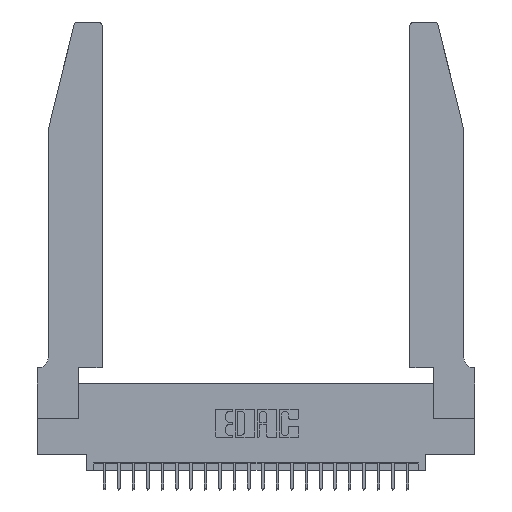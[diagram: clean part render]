
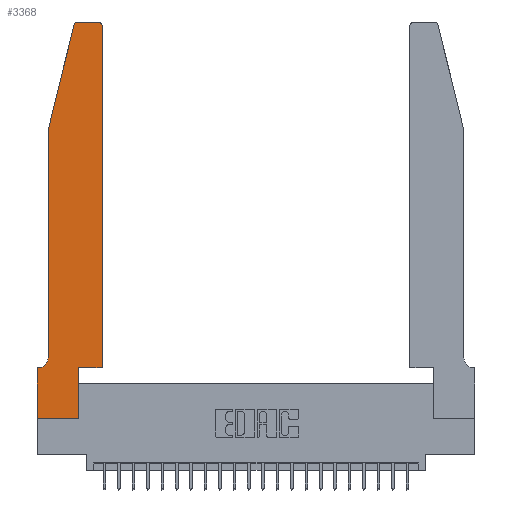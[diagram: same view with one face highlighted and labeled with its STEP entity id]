
A CAD part, top view. The second image highlights one B-rep face of the part: STEP entity #3368.
In plain terms, the highlighted planar face has unit normal (0, 0, 1).
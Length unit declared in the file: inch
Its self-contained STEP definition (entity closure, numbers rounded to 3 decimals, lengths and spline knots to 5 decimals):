
#130 = DIRECTION ( 'NONE',  ( -0.239, -0.971, 0. ) ) ;
#488 = CARTESIAN_POINT ( 'NONE',  ( 0.0755, 2., 0.37 ) ) ;
#593 = EDGE_CURVE ( 'NONE', #7490, #12814, #12112, .T. ) ;
#648 = DIRECTION ( 'NONE',  ( 1., 0., 0. ) ) ;
#913 = EDGE_CURVE ( 'NONE', #7336, #8099, #11092, .T. ) ;
#1111 = DIRECTION ( 'NONE',  ( 0., 0., 1. ) ) ;
#1281 = CARTESIAN_POINT ( 'NONE',  ( 0.0755, 0.42, 0.37 ) ) ;
#1291 = ORIENTED_EDGE ( 'NONE', *, *, #3324, .T. ) ;
#1576 = ORIENTED_EDGE ( 'NONE', *, *, #6813, .T. ) ;
#1815 = CIRCLE ( 'NONE', #7469, 0.07 ) ;
#1848 = ORIENTED_EDGE ( 'NONE', *, *, #8967, .T. ) ;
#2276 = VERTEX_POINT ( 'NONE', #1281 ) ;
#2539 = CARTESIAN_POINT ( 'NONE',  ( 0.2605, 2.75, 0.37 ) ) ;
#2674 = DIRECTION ( 'NONE',  ( -1., 0., 0. ) ) ;
#2906 = CIRCLE ( 'NONE', #4933, 0.03 ) ;
#3324 = EDGE_CURVE ( 'NONE', #22680, #20967, #6829, .T. ) ;
#3368 = ADVANCED_FACE ( 'NONE', ( #19996 ), #8461, .T. ) ;
#3487 = LINE ( 'NONE', #17595, #19776 ) ;
#3553 = DIRECTION ( 'NONE',  ( 0., 0., 1. ) ) ;
#4190 = EDGE_CURVE ( 'NONE', #8099, #7490, #8575, .T. ) ;
#4331 = CARTESIAN_POINT ( 'NONE',  ( 0.284, 2.75, 0.37 ) ) ;
#4577 = VECTOR ( 'NONE', #10924, 39.37008 ) ;
#4749 = CARTESIAN_POINT ( 'NONE',  ( 0., 0.35, 0.37 ) ) ;
#4921 = CARTESIAN_POINT ( 'NONE',  ( 0.284, 2.72, 0.37 ) ) ;
#4933 = AXIS2_PLACEMENT_3D ( 'NONE', #4921, #5051, #648 ) ;
#5051 = DIRECTION ( 'NONE',  ( 0., 0., 1. ) ) ;
#5195 = CARTESIAN_POINT ( 'NONE',  ( 0., 0.35, 0.37 ) ) ;
#5705 = DIRECTION ( 'NONE',  ( 1., 0., 0. ) ) ;
#6469 = CARTESIAN_POINT ( 'NONE',  ( 0.4505, 0.35, 0.37 ) ) ;
#6543 = EDGE_LOOP ( 'NONE', ( #20615, #11141, #1848, #9498, #13124, #1291, #6877, #1576, #17519, #9753, #21672, #21917 ) ) ;
#6564 = AXIS2_PLACEMENT_3D ( 'NONE', #5195, #3553, #5705 ) ;
#6805 = CARTESIAN_POINT ( 'NONE',  ( 0.25487, 2.72718, 0.37 ) ) ;
#6813 = EDGE_CURVE ( 'NONE', #21312, #22938, #16351, .T. ) ;
#6829 = LINE ( 'NONE', #12498, #7353 ) ;
#6877 = ORIENTED_EDGE ( 'NONE', *, *, #10868, .T. ) ;
#6899 = CARTESIAN_POINT ( 'NONE',  ( 0.4205, 2.72, 0.37 ) ) ;
#7044 = VECTOR ( 'NONE', #22953, 39.37008 ) ;
#7259 = VECTOR ( 'NONE', #21099, 39.37008 ) ;
#7336 = VERTEX_POINT ( 'NONE', #6469 ) ;
#7353 = VECTOR ( 'NONE', #2674, 39.37008 ) ;
#7469 = AXIS2_PLACEMENT_3D ( 'NONE', #24534, #11494, #19239 ) ;
#7490 = VERTEX_POINT ( 'NONE', #19339 ) ;
#7692 = EDGE_CURVE ( 'NONE', #12814, #21401, #2906, .T. ) ;
#8016 = VERTEX_POINT ( 'NONE', #488 ) ;
#8047 = CARTESIAN_POINT ( 'NONE',  ( 0., 0., 0.37 ) ) ;
#8099 = VERTEX_POINT ( 'NONE', #9552 ) ;
#8461 = PLANE ( 'NONE',  #6564 ) ;
#8575 = CIRCLE ( 'NONE', #22724, 0.03 ) ;
#8862 = DIRECTION ( 'NONE',  ( 1., 0., 0. ) ) ;
#8967 = EDGE_CURVE ( 'NONE', #21401, #8016, #13976, .T. ) ;
#9155 = LINE ( 'NONE', #22331, #4577 ) ;
#9498 = ORIENTED_EDGE ( 'NONE', *, *, #13489, .T. ) ;
#9552 = CARTESIAN_POINT ( 'NONE',  ( 0.4505, 2.72, 0.37 ) ) ;
#9753 = ORIENTED_EDGE ( 'NONE', *, *, #18154, .T. ) ;
#10868 = EDGE_CURVE ( 'NONE', #20967, #21312, #21610, .T. ) ;
#10924 = DIRECTION ( 'NONE',  ( 0., -1., 0. ) ) ;
#11092 = LINE ( 'NONE', #22988, #7259 ) ;
#11141 = ORIENTED_EDGE ( 'NONE', *, *, #7692, .T. ) ;
#11494 = DIRECTION ( 'NONE',  ( 0., 0., -1. ) ) ;
#11548 = EDGE_CURVE ( 'NONE', #2276, #22680, #1815, .T. ) ;
#11661 = CARTESIAN_POINT ( 'NONE',  ( 0.2865, 0.35, 0.37 ) ) ;
#12112 = LINE ( 'NONE', #2539, #20570 ) ;
#12498 = CARTESIAN_POINT ( 'NONE',  ( 0.0755, 0.35, 0.37 ) ) ;
#12613 = VERTEX_POINT ( 'NONE', #14082 ) ;
#12768 = CARTESIAN_POINT ( 'NONE',  ( 0., 0., 0.37 ) ) ;
#12814 = VERTEX_POINT ( 'NONE', #4331 ) ;
#13124 = ORIENTED_EDGE ( 'NONE', *, *, #11548, .T. ) ;
#13489 = EDGE_CURVE ( 'NONE', #8016, #2276, #9155, .T. ) ;
#13524 = DIRECTION ( 'NONE',  ( 1., 0., 0. ) ) ;
#13976 = LINE ( 'NONE', #15389, #17085 ) ;
#14082 = CARTESIAN_POINT ( 'NONE',  ( 0.2865, 0.35, 0.37 ) ) ;
#14724 = DIRECTION ( 'NONE',  ( 1., 0., 0. ) ) ;
#14889 = EDGE_CURVE ( 'NONE', #22938, #12613, #15236, .T. ) ;
#15236 = LINE ( 'NONE', #11661, #7044 ) ;
#15389 = CARTESIAN_POINT ( 'NONE',  ( 0.0755, 2., 0.37 ) ) ;
#15776 = DIRECTION ( 'NONE',  ( 0., -1., 0. ) ) ;
#16351 = LINE ( 'NONE', #12768, #16604 ) ;
#16604 = VECTOR ( 'NONE', #8862, 39.37008 ) ;
#17085 = VECTOR ( 'NONE', #130, 39.37008 ) ;
#17519 = ORIENTED_EDGE ( 'NONE', *, *, #14889, .T. ) ;
#17595 = CARTESIAN_POINT ( 'NONE',  ( 0.4505, 0.35, 0.37 ) ) ;
#18096 = CARTESIAN_POINT ( 'NONE',  ( 0.0055, 0.35, 0.37 ) ) ;
#18154 = EDGE_CURVE ( 'NONE', #12613, #7336, #3487, .T. ) ;
#19239 = DIRECTION ( 'NONE',  ( -1., 0., 0. ) ) ;
#19339 = CARTESIAN_POINT ( 'NONE',  ( 0.4205, 2.75, 0.37 ) ) ;
#19776 = VECTOR ( 'NONE', #13524, 39.37008 ) ;
#19996 = FACE_OUTER_BOUND ( 'NONE', #6543, .T. ) ;
#20570 = VECTOR ( 'NONE', #21635, 39.37008 ) ;
#20615 = ORIENTED_EDGE ( 'NONE', *, *, #593, .T. ) ;
#20967 = VERTEX_POINT ( 'NONE', #4749 ) ;
#21099 = DIRECTION ( 'NONE',  ( 0., 1., 0. ) ) ;
#21312 = VERTEX_POINT ( 'NONE', #23289 ) ;
#21401 = VERTEX_POINT ( 'NONE', #6805 ) ;
#21587 = VECTOR ( 'NONE', #15776, 39.37008 ) ;
#21610 = LINE ( 'NONE', #8047, #21587 ) ;
#21628 = CARTESIAN_POINT ( 'NONE',  ( 0.2865, 0., 0.37 ) ) ;
#21635 = DIRECTION ( 'NONE',  ( -1., 0., 0. ) ) ;
#21672 = ORIENTED_EDGE ( 'NONE', *, *, #913, .T. ) ;
#21917 = ORIENTED_EDGE ( 'NONE', *, *, #4190, .T. ) ;
#22331 = CARTESIAN_POINT ( 'NONE',  ( 0.0755, 2., 0.37 ) ) ;
#22680 = VERTEX_POINT ( 'NONE', #18096 ) ;
#22724 = AXIS2_PLACEMENT_3D ( 'NONE', #6899, #1111, #14724 ) ;
#22938 = VERTEX_POINT ( 'NONE', #21628 ) ;
#22953 = DIRECTION ( 'NONE',  ( 0., 1., 0. ) ) ;
#22988 = CARTESIAN_POINT ( 'NONE',  ( 0.4505, 0.35, 0.37 ) ) ;
#23289 = CARTESIAN_POINT ( 'NONE',  ( 0., 0., 0.37 ) ) ;
#24534 = CARTESIAN_POINT ( 'NONE',  ( 0.0055, 0.42, 0.37 ) ) ;
